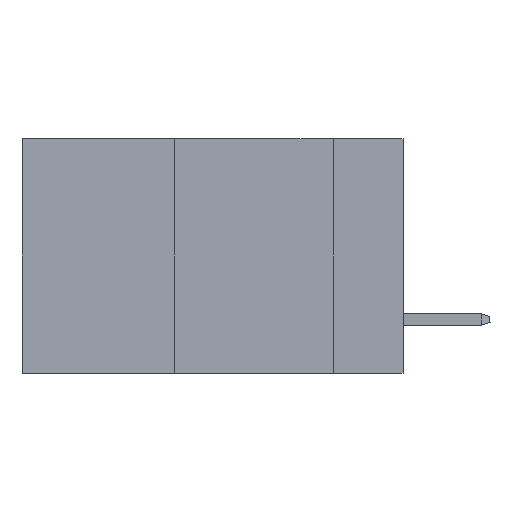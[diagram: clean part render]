
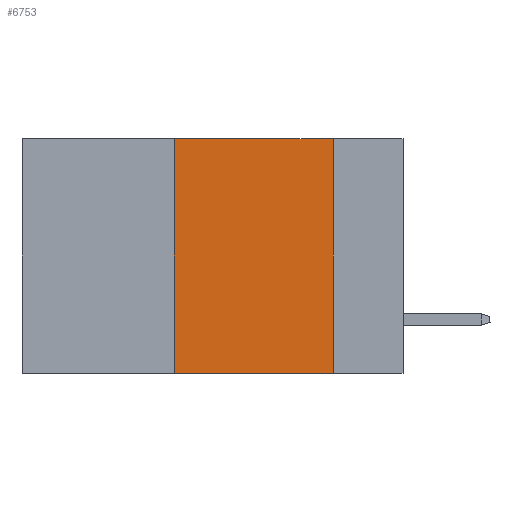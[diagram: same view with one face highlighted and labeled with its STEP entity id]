
A CAD part, left-side view. The second image highlights one B-rep face of the part: STEP entity #6753.
In plain terms, the highlighted planar face has unit normal (-1, 0, 0).
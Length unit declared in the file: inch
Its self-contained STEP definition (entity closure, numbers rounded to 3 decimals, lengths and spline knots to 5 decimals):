
#2837 = VECTOR ( 'NONE', #5566, 39.37008 ) ;
#3215 = VERTEX_POINT ( 'NONE', #37217 ) ;
#5566 = DIRECTION ( 'NONE',  ( 0., 0., 1. ) ) ;
#5579 = LINE ( 'NONE', #18242, #14940 ) ;
#5592 = LINE ( 'NONE', #40902, #23950 ) ;
#6753 = ADVANCED_FACE ( 'NONE', ( #31788 ), #18692, .F. ) ;
#7233 = ORIENTED_EDGE ( 'NONE', *, *, #26558, .F. ) ;
#9100 = LINE ( 'NONE', #21752, #2837 ) ;
#11318 = VERTEX_POINT ( 'NONE', #17017 ) ;
#12068 = CARTESIAN_POINT ( 'NONE',  ( 0., 0.6, 0. ) ) ;
#12707 = EDGE_CURVE ( 'NONE', #24600, #26373, #5579, .T. ) ;
#13346 = ORIENTED_EDGE ( 'NONE', *, *, #36975, .F. ) ;
#14702 = DIRECTION ( 'NONE',  ( 0., -1., 0. ) ) ;
#14940 = VECTOR ( 'NONE', #14702, 39.37008 ) ;
#16990 = ORIENTED_EDGE ( 'NONE', *, *, #36280, .T. ) ;
#17017 = CARTESIAN_POINT ( 'NONE',  ( 0., 0.11, -0.37 ) ) ;
#17318 = DIRECTION ( 'NONE',  ( 0., 0., -1. ) ) ;
#18242 = CARTESIAN_POINT ( 'NONE',  ( 0., 0.6, 0. ) ) ;
#18692 = PLANE ( 'NONE',  #31530 ) ;
#20445 = EDGE_LOOP ( 'NONE', ( #13346, #27369, #7233, #16990 ) ) ;
#21752 = CARTESIAN_POINT ( 'NONE',  ( 0., 0.36, 0. ) ) ;
#23950 = VECTOR ( 'NONE', #30943, 39.37008 ) ;
#24600 = VERTEX_POINT ( 'NONE', #25797 ) ;
#25797 = CARTESIAN_POINT ( 'NONE',  ( 0., 0.36, 0. ) ) ;
#26373 = VERTEX_POINT ( 'NONE', #39646 ) ;
#26558 = EDGE_CURVE ( 'NONE', #3215, #24600, #9100, .T. ) ;
#27369 = ORIENTED_EDGE ( 'NONE', *, *, #12707, .F. ) ;
#28006 = VECTOR ( 'NONE', #17318, 39.37008 ) ;
#29411 = CARTESIAN_POINT ( 'NONE',  ( 0., 0.11, 0. ) ) ;
#30943 = DIRECTION ( 'NONE',  ( 0., -1., 0. ) ) ;
#31530 = AXIS2_PLACEMENT_3D ( 'NONE', #12068, #37821, #31597 ) ;
#31597 = DIRECTION ( 'NONE',  ( 0., 0., -1. ) ) ;
#31788 = FACE_OUTER_BOUND ( 'NONE', #20445, .T. ) ;
#36280 = EDGE_CURVE ( 'NONE', #3215, #11318, #5592, .T. ) ;
#36975 = EDGE_CURVE ( 'NONE', #26373, #11318, #39576, .T. ) ;
#37217 = CARTESIAN_POINT ( 'NONE',  ( 0., 0.36, -0.37 ) ) ;
#37821 = DIRECTION ( 'NONE',  ( 1., 0., 0. ) ) ;
#39576 = LINE ( 'NONE', #29411, #28006 ) ;
#39646 = CARTESIAN_POINT ( 'NONE',  ( 0., 0.11, 0. ) ) ;
#40902 = CARTESIAN_POINT ( 'NONE',  ( 0., 0.6, -0.37 ) ) ;
